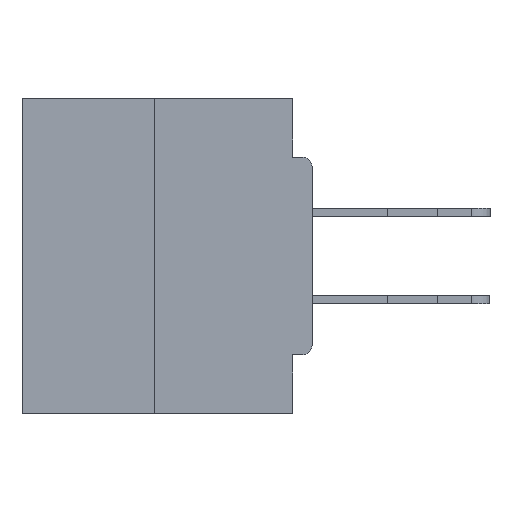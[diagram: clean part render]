
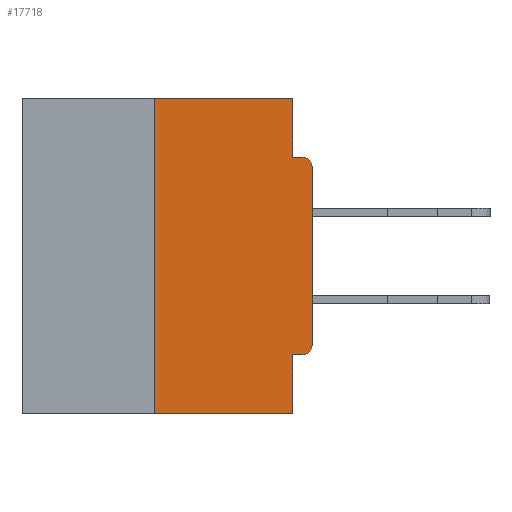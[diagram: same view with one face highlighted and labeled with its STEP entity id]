
A CAD part, left-side view. The second image highlights one B-rep face of the part: STEP entity #17718.
In plain terms, the highlighted planar face has unit normal (-1, 0, 0).
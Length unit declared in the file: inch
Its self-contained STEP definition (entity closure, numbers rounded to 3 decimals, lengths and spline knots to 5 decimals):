
#503 = DIRECTION ( 'NONE',  ( 0., 0., 1. ) ) ;
#1783 = CARTESIAN_POINT ( 'NONE',  ( 0., 0.031, -0.4065 ) ) ;
#2233 = DIRECTION ( 'NONE',  ( 0., 0., -1. ) ) ;
#3324 = EDGE_CURVE ( 'NONE', #6873, #32039, #26379, .T. ) ;
#3373 = FACE_OUTER_BOUND ( 'NONE', #17683, .T. ) ;
#4781 = EDGE_CURVE ( 'NONE', #22731, #9606, #13202, .T. ) ;
#4831 = VERTEX_POINT ( 'NONE', #21834 ) ;
#5069 = ORIENTED_EDGE ( 'NONE', *, *, #6666, .F. ) ;
#5880 = ORIENTED_EDGE ( 'NONE', *, *, #15199, .F. ) ;
#6666 = EDGE_CURVE ( 'NONE', #4831, #31605, #29555, .T. ) ;
#6772 = DIRECTION ( 'NONE',  ( 0., 0., -1. ) ) ;
#6873 = VERTEX_POINT ( 'NONE', #27199 ) ;
#7292 = CARTESIAN_POINT ( 'NONE',  ( 0., 0.031, -0.0935 ) ) ;
#7645 = VECTOR ( 'NONE', #21281, 39.37008 ) ;
#8202 = CARTESIAN_POINT ( 'NONE',  ( 0., 0.031, -0.5 ) ) ;
#8297 = VECTOR ( 'NONE', #503, 39.37008 ) ;
#8510 = DIRECTION ( 'NONE',  ( 0., -1., 0. ) ) ;
#8844 = VECTOR ( 'NONE', #8510, 39.37008 ) ;
#8876 = CARTESIAN_POINT ( 'NONE',  ( 0., 0.031, 0. ) ) ;
#9121 = CARTESIAN_POINT ( 'NONE',  ( 0., 0.015, -0.0935 ) ) ;
#9313 = LINE ( 'NONE', #20297, #13895 ) ;
#9502 = VERTEX_POINT ( 'NONE', #8876 ) ;
#9606 = VERTEX_POINT ( 'NONE', #21855 ) ;
#9957 = LINE ( 'NONE', #22715, #11158 ) ;
#10698 = CARTESIAN_POINT ( 'NONE',  ( 0., 0., -0.0935 ) ) ;
#10703 = CARTESIAN_POINT ( 'NONE',  ( 0., 0.46, 0. ) ) ;
#11115 = VECTOR ( 'NONE', #15859, 39.37008 ) ;
#11158 = VECTOR ( 'NONE', #2233, 39.37008 ) ;
#11604 = CARTESIAN_POINT ( 'NONE',  ( 0., 0., -0.3915 ) ) ;
#11635 = VERTEX_POINT ( 'NONE', #7292 ) ;
#12015 = CARTESIAN_POINT ( 'NONE',  ( 0., 0.25, 0. ) ) ;
#12179 = EDGE_CURVE ( 'NONE', #9502, #11635, #9313, .T. ) ;
#12862 = ORIENTED_EDGE ( 'NONE', *, *, #32839, .F. ) ;
#13115 = CARTESIAN_POINT ( 'NONE',  ( 0., 0., 0. ) ) ;
#13202 = LINE ( 'NONE', #13115, #14927 ) ;
#13227 = ORIENTED_EDGE ( 'NONE', *, *, #3324, .F. ) ;
#13665 = EDGE_CURVE ( 'NONE', #4831, #22731, #17603, .T. ) ;
#13895 = VECTOR ( 'NONE', #28280, 39.37008 ) ;
#14665 = CARTESIAN_POINT ( 'NONE',  ( 0., 0.015, -0.3915 ) ) ;
#14927 = VECTOR ( 'NONE', #18673, 39.37008 ) ;
#15199 = EDGE_CURVE ( 'NONE', #31605, #15454, #9957, .T. ) ;
#15454 = VERTEX_POINT ( 'NONE', #8202 ) ;
#15655 = ORIENTED_EDGE ( 'NONE', *, *, #33686, .F. ) ;
#15859 = DIRECTION ( 'NONE',  ( 0., -1., 0. ) ) ;
#17153 = ORIENTED_EDGE ( 'NONE', *, *, #23672, .T. ) ;
#17603 = CIRCLE ( 'NONE', #32432, 0.015 ) ;
#17683 = EDGE_LOOP ( 'NONE', ( #15655, #13227, #18742, #5880, #5069, #20852, #27011, #17153, #12862, #21967 ) ) ;
#17718 = ADVANCED_FACE ( 'NONE', ( #3373 ), #24343, .F. ) ;
#18673 = DIRECTION ( 'NONE',  ( 0., 0., 1. ) ) ;
#18742 = ORIENTED_EDGE ( 'NONE', *, *, #32016, .T. ) ;
#19087 = DIRECTION ( 'NONE',  ( 0., 0., -1. ) ) ;
#19869 = LINE ( 'NONE', #34091, #7645 ) ;
#20297 = CARTESIAN_POINT ( 'NONE',  ( 0., 0.031, 0. ) ) ;
#20852 = ORIENTED_EDGE ( 'NONE', *, *, #13665, .T. ) ;
#21267 = AXIS2_PLACEMENT_3D ( 'NONE', #10703, #23877, #32219 ) ;
#21281 = DIRECTION ( 'NONE',  ( 0., -1., 0. ) ) ;
#21531 = VERTEX_POINT ( 'NONE', #9121 ) ;
#21834 = CARTESIAN_POINT ( 'NONE',  ( 0., 0.015, -0.4065 ) ) ;
#21855 = CARTESIAN_POINT ( 'NONE',  ( 0., 0., -0.1085 ) ) ;
#21967 = ORIENTED_EDGE ( 'NONE', *, *, #12179, .F. ) ;
#22566 = DIRECTION ( 'NONE',  ( 0., 1., 0. ) ) ;
#22687 = CARTESIAN_POINT ( 'NONE',  ( 0., 0., -0.4065 ) ) ;
#22715 = CARTESIAN_POINT ( 'NONE',  ( 0., 0.031, -0.5 ) ) ;
#22731 = VERTEX_POINT ( 'NONE', #11604 ) ;
#22992 = CIRCLE ( 'NONE', #25704, 0.015 ) ;
#23257 = VECTOR ( 'NONE', #22566, 39.37008 ) ;
#23672 = EDGE_CURVE ( 'NONE', #9606, #21531, #22992, .T. ) ;
#23877 = DIRECTION ( 'NONE',  ( 1., 0., 0. ) ) ;
#24343 = PLANE ( 'NONE',  #21267 ) ;
#24634 = CARTESIAN_POINT ( 'NONE',  ( 0., 0.46, -0.5 ) ) ;
#25704 = AXIS2_PLACEMENT_3D ( 'NONE', #29703, #27075, #19087 ) ;
#26379 = LINE ( 'NONE', #30232, #8297 ) ;
#27011 = ORIENTED_EDGE ( 'NONE', *, *, #4781, .T. ) ;
#27075 = DIRECTION ( 'NONE',  ( -1., 0., 0. ) ) ;
#27199 = CARTESIAN_POINT ( 'NONE',  ( 0., 0.25, -0.5 ) ) ;
#28280 = DIRECTION ( 'NONE',  ( 0., 0., -1. ) ) ;
#28573 = DIRECTION ( 'NONE',  ( -1., 0., 0. ) ) ;
#29555 = LINE ( 'NONE', #22687, #23257 ) ;
#29703 = CARTESIAN_POINT ( 'NONE',  ( 0., 0.015, -0.1085 ) ) ;
#30232 = CARTESIAN_POINT ( 'NONE',  ( 0., 0.25, 0. ) ) ;
#31605 = VERTEX_POINT ( 'NONE', #1783 ) ;
#31622 = LINE ( 'NONE', #24634, #8844 ) ;
#32016 = EDGE_CURVE ( 'NONE', #6873, #15454, #31622, .T. ) ;
#32039 = VERTEX_POINT ( 'NONE', #12015 ) ;
#32219 = DIRECTION ( 'NONE',  ( 0., 0., -1. ) ) ;
#32432 = AXIS2_PLACEMENT_3D ( 'NONE', #14665, #28573, #6772 ) ;
#32839 = EDGE_CURVE ( 'NONE', #11635, #21531, #34692, .T. ) ;
#33686 = EDGE_CURVE ( 'NONE', #32039, #9502, #19869, .T. ) ;
#34091 = CARTESIAN_POINT ( 'NONE',  ( 0., 0.46, 0. ) ) ;
#34692 = LINE ( 'NONE', #10698, #11115 ) ;
